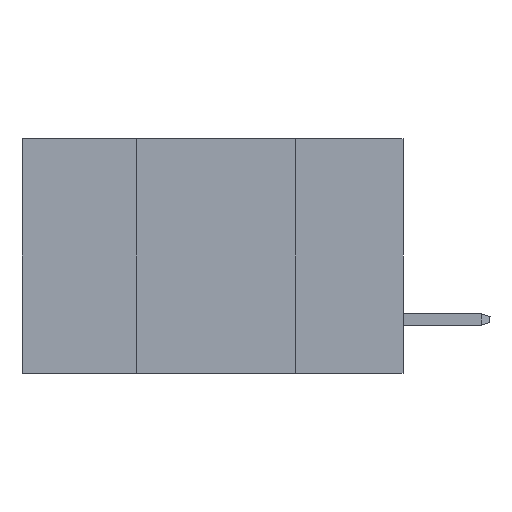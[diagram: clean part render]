
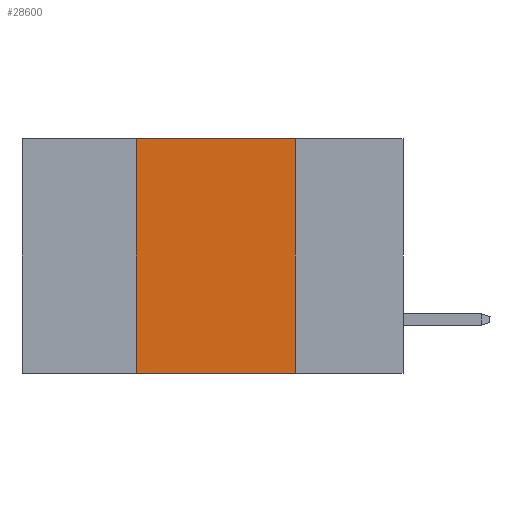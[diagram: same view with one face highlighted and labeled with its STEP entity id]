
A CAD part, left-side view. The second image highlights one B-rep face of the part: STEP entity #28600.
In plain terms, the highlighted planar face has unit normal (-1, 0, 0).
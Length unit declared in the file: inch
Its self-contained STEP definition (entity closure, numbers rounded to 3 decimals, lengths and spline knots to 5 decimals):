
#2170 = EDGE_CURVE ( 'NONE', #12946, #8607, #3183, .T. ) ;
#2528 = LINE ( 'NONE', #8470, #11361 ) ;
#2796 = CARTESIAN_POINT ( 'NONE',  ( 0., 0.17, 0. ) ) ;
#3183 = LINE ( 'NONE', #14903, #26254 ) ;
#3821 = EDGE_CURVE ( 'NONE', #21984, #14805, #2528, .T. ) ;
#4271 = VECTOR ( 'NONE', #14166, 39.37008 ) ;
#5518 = VECTOR ( 'NONE', #21144, 39.37008 ) ;
#6550 = FACE_OUTER_BOUND ( 'NONE', #25895, .T. ) ;
#8386 = CARTESIAN_POINT ( 'NONE',  ( 0., 0.6, -0.37 ) ) ;
#8470 = CARTESIAN_POINT ( 'NONE',  ( 0., 0.17, 0. ) ) ;
#8607 = VERTEX_POINT ( 'NONE', #25767 ) ;
#9647 = DIRECTION ( 'NONE',  ( 1., 0., 0. ) ) ;
#10210 = DIRECTION ( 'NONE',  ( 0., 0., -1. ) ) ;
#10671 = EDGE_CURVE ( 'NONE', #12946, #14805, #14356, .T. ) ;
#10840 = AXIS2_PLACEMENT_3D ( 'NONE', #33471, #9647, #10210 ) ;
#11153 = EDGE_CURVE ( 'NONE', #8607, #21984, #18262, .T. ) ;
#11361 = VECTOR ( 'NONE', #20176, 39.37008 ) ;
#12005 = DIRECTION ( 'NONE',  ( 0., 0., 1. ) ) ;
#12946 = VERTEX_POINT ( 'NONE', #26863 ) ;
#14166 = DIRECTION ( 'NONE',  ( 0., -1., 0. ) ) ;
#14356 = LINE ( 'NONE', #8386, #4271 ) ;
#14805 = VERTEX_POINT ( 'NONE', #25334 ) ;
#14903 = CARTESIAN_POINT ( 'NONE',  ( 0., 0.42, 0. ) ) ;
#15251 = ORIENTED_EDGE ( 'NONE', *, *, #2170, .F. ) ;
#18262 = LINE ( 'NONE', #27287, #5518 ) ;
#20176 = DIRECTION ( 'NONE',  ( 0., 0., -1. ) ) ;
#21144 = DIRECTION ( 'NONE',  ( 0., -1., 0. ) ) ;
#21734 = PLANE ( 'NONE',  #10840 ) ;
#21984 = VERTEX_POINT ( 'NONE', #2796 ) ;
#24836 = ORIENTED_EDGE ( 'NONE', *, *, #11153, .F. ) ;
#25334 = CARTESIAN_POINT ( 'NONE',  ( 0., 0.17, -0.37 ) ) ;
#25767 = CARTESIAN_POINT ( 'NONE',  ( 0., 0.42, 0. ) ) ;
#25895 = EDGE_LOOP ( 'NONE', ( #27591, #24836, #15251, #29900 ) ) ;
#26254 = VECTOR ( 'NONE', #12005, 39.37008 ) ;
#26863 = CARTESIAN_POINT ( 'NONE',  ( 0., 0.42, -0.37 ) ) ;
#27287 = CARTESIAN_POINT ( 'NONE',  ( 0., 0.6, 0. ) ) ;
#27591 = ORIENTED_EDGE ( 'NONE', *, *, #3821, .F. ) ;
#28600 = ADVANCED_FACE ( 'NONE', ( #6550 ), #21734, .F. ) ;
#29900 = ORIENTED_EDGE ( 'NONE', *, *, #10671, .T. ) ;
#33471 = CARTESIAN_POINT ( 'NONE',  ( 0., 0.6, 0. ) ) ;
